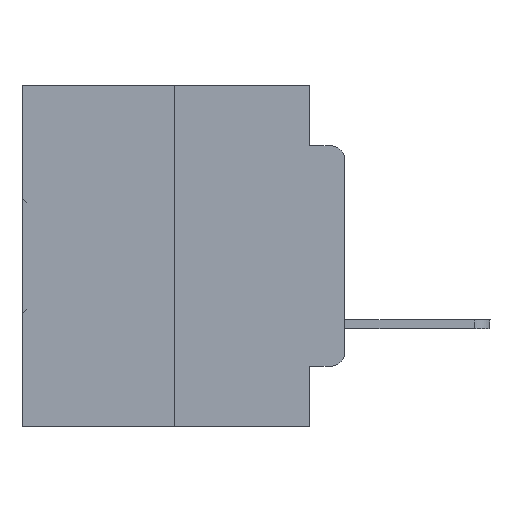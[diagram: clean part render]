
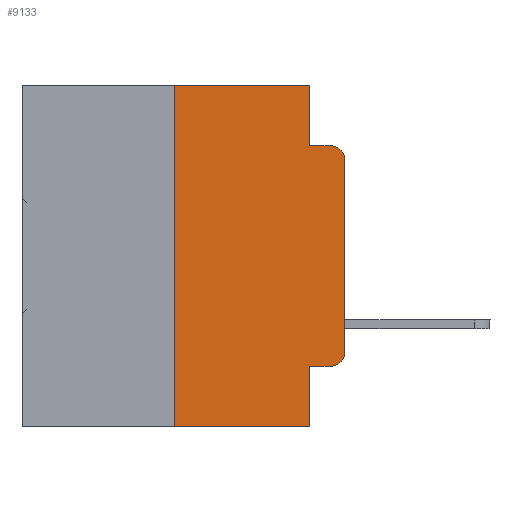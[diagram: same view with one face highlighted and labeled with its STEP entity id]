
A CAD part, left-side view. The second image highlights one B-rep face of the part: STEP entity #9133.
In plain terms, the highlighted planar face has unit normal (-1, 0, 0).
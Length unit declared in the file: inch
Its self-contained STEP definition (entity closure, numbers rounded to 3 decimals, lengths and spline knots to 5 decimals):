
#59 = DIRECTION ( 'NONE',  ( -1., 0., 0. ) ) ;
#85 = VERTEX_POINT ( 'NONE', #13878 ) ;
#726 = VECTOR ( 'NONE', #14257, 39.37008 ) ;
#1128 = ORIENTED_EDGE ( 'NONE', *, *, #7032, .T. ) ;
#1382 = CARTESIAN_POINT ( 'NONE',  ( 0., 0.051, -0.0885 ) ) ;
#2603 = VERTEX_POINT ( 'NONE', #13862 ) ;
#2718 = DIRECTION ( 'NONE',  ( -1., 0., 0. ) ) ;
#3295 = EDGE_CURVE ( 'NONE', #10744, #25735, #5324, .T. ) ;
#3365 = AXIS2_PLACEMENT_3D ( 'NONE', #13072, #2718, #13231 ) ;
#3642 = VERTEX_POINT ( 'NONE', #25861 ) ;
#3797 = ORIENTED_EDGE ( 'NONE', *, *, #25758, .T. ) ;
#4208 = ORIENTED_EDGE ( 'NONE', *, *, #4446, .F. ) ;
#4446 = EDGE_CURVE ( 'NONE', #7122, #23000, #22796, .T. ) ;
#4670 = DIRECTION ( 'NONE',  ( 0., 0., -1. ) ) ;
#5116 = VECTOR ( 'NONE', #30792, 39.37008 ) ;
#5136 = VECTOR ( 'NONE', #8825, 39.37008 ) ;
#5295 = DIRECTION ( 'NONE',  ( 0., -1., 0. ) ) ;
#5324 = LINE ( 'NONE', #10666, #18778 ) ;
#5916 = CARTESIAN_POINT ( 'NONE',  ( 0., 0.051, 0. ) ) ;
#6122 = DIRECTION ( 'NONE',  ( 0., -1., 0. ) ) ;
#6758 = CARTESIAN_POINT ( 'NONE',  ( 0., 0.051, -0.4115 ) ) ;
#7032 = EDGE_CURVE ( 'NONE', #85, #11149, #7097, .T. ) ;
#7097 = LINE ( 'NONE', #6758, #33223 ) ;
#7122 = VERTEX_POINT ( 'NONE', #20211 ) ;
#7894 = ORIENTED_EDGE ( 'NONE', *, *, #12484, .F. ) ;
#8657 = LINE ( 'NONE', #1382, #5136 ) ;
#8685 = ORIENTED_EDGE ( 'NONE', *, *, #3295, .T. ) ;
#8825 = DIRECTION ( 'NONE',  ( 0., -1., 0. ) ) ;
#8903 = EDGE_CURVE ( 'NONE', #23000, #2603, #8657, .T. ) ;
#9133 = ADVANCED_FACE ( 'NONE', ( #17783 ), #28354, .F. ) ;
#9675 = EDGE_CURVE ( 'NONE', #29108, #7122, #23612, .T. ) ;
#10666 = CARTESIAN_POINT ( 'NONE',  ( 0., 0.473, -0.5 ) ) ;
#10744 = VERTEX_POINT ( 'NONE', #33350 ) ;
#11149 = VERTEX_POINT ( 'NONE', #25227 ) ;
#12217 = DIRECTION ( 'NONE',  ( 0., 0., 1. ) ) ;
#12484 = EDGE_CURVE ( 'NONE', #85, #25735, #16612, .T. ) ;
#12672 = CIRCLE ( 'NONE', #34238, 0.02 ) ;
#13072 = CARTESIAN_POINT ( 'NONE',  ( 0., 0.02, -0.1085 ) ) ;
#13231 = DIRECTION ( 'NONE',  ( 0., 0., -1. ) ) ;
#13820 = DIRECTION ( 'NONE',  ( 0., 0., -1. ) ) ;
#13862 = CARTESIAN_POINT ( 'NONE',  ( 0., 0.02, -0.0885 ) ) ;
#13878 = CARTESIAN_POINT ( 'NONE',  ( 0., 0.051, -0.4115 ) ) ;
#14257 = DIRECTION ( 'NONE',  ( 0., 0., 1. ) ) ;
#14267 = CARTESIAN_POINT ( 'NONE',  ( 0., 0.25, 0. ) ) ;
#15153 = CARTESIAN_POINT ( 'NONE',  ( 0., 0.473, 0. ) ) ;
#15179 = CARTESIAN_POINT ( 'NONE',  ( 0., 0., -0.1085 ) ) ;
#15857 = DIRECTION ( 'NONE',  ( 0., -1., 0. ) ) ;
#16612 = LINE ( 'NONE', #5916, #31786 ) ;
#17286 = EDGE_LOOP ( 'NONE', ( #3797, #25027, #24393, #4208, #22841, #23586, #8685, #7894, #1128, #25691 ) ) ;
#17783 = FACE_OUTER_BOUND ( 'NONE', #17286, .T. ) ;
#18042 = CARTESIAN_POINT ( 'NONE',  ( 0., 0.051, -0.0885 ) ) ;
#18778 = VECTOR ( 'NONE', #15857, 39.37008 ) ;
#18804 = CIRCLE ( 'NONE', #3365, 0.02 ) ;
#18873 = EDGE_CURVE ( 'NONE', #11149, #3642, #12672, .T. ) ;
#18953 = VECTOR ( 'NONE', #5295, 39.37008 ) ;
#19025 = CARTESIAN_POINT ( 'NONE',  ( 0., 0., 0. ) ) ;
#20066 = VERTEX_POINT ( 'NONE', #15179 ) ;
#20186 = EDGE_CURVE ( 'NONE', #20066, #2603, #18804, .T. ) ;
#20211 = CARTESIAN_POINT ( 'NONE',  ( 0., 0.051, 0. ) ) ;
#20539 = DIRECTION ( 'NONE',  ( 1., 0., 0. ) ) ;
#20718 = CARTESIAN_POINT ( 'NONE',  ( 0., 0.473, 0. ) ) ;
#22796 = LINE ( 'NONE', #30963, #5116 ) ;
#22841 = ORIENTED_EDGE ( 'NONE', *, *, #9675, .F. ) ;
#23000 = VERTEX_POINT ( 'NONE', #18042 ) ;
#23127 = DIRECTION ( 'NONE',  ( 0., 0., -1. ) ) ;
#23586 = ORIENTED_EDGE ( 'NONE', *, *, #23887, .F. ) ;
#23612 = LINE ( 'NONE', #15153, #18953 ) ;
#23887 = EDGE_CURVE ( 'NONE', #10744, #29108, #30212, .T. ) ;
#24393 = ORIENTED_EDGE ( 'NONE', *, *, #8903, .F. ) ;
#24997 = AXIS2_PLACEMENT_3D ( 'NONE', #20718, #20539, #4670 ) ;
#25027 = ORIENTED_EDGE ( 'NONE', *, *, #20186, .T. ) ;
#25227 = CARTESIAN_POINT ( 'NONE',  ( 0., 0.02, -0.4115 ) ) ;
#25433 = VECTOR ( 'NONE', #12217, 39.37008 ) ;
#25691 = ORIENTED_EDGE ( 'NONE', *, *, #18873, .T. ) ;
#25735 = VERTEX_POINT ( 'NONE', #32391 ) ;
#25758 = EDGE_CURVE ( 'NONE', #3642, #20066, #26818, .T. ) ;
#25861 = CARTESIAN_POINT ( 'NONE',  ( 0., 0., -0.3915 ) ) ;
#26729 = CARTESIAN_POINT ( 'NONE',  ( 0., 0.25, 0. ) ) ;
#26818 = LINE ( 'NONE', #19025, #25433 ) ;
#28354 = PLANE ( 'NONE',  #24997 ) ;
#29108 = VERTEX_POINT ( 'NONE', #14267 ) ;
#29306 = CARTESIAN_POINT ( 'NONE',  ( 0., 0.02, -0.3915 ) ) ;
#30212 = LINE ( 'NONE', #26729, #726 ) ;
#30792 = DIRECTION ( 'NONE',  ( 0., 0., -1. ) ) ;
#30963 = CARTESIAN_POINT ( 'NONE',  ( 0., 0.051, 0. ) ) ;
#31786 = VECTOR ( 'NONE', #13820, 39.37008 ) ;
#32391 = CARTESIAN_POINT ( 'NONE',  ( 0., 0.051, -0.5 ) ) ;
#33223 = VECTOR ( 'NONE', #6122, 39.37008 ) ;
#33350 = CARTESIAN_POINT ( 'NONE',  ( 0., 0.25, -0.5 ) ) ;
#34238 = AXIS2_PLACEMENT_3D ( 'NONE', #29306, #59, #23127 ) ;
